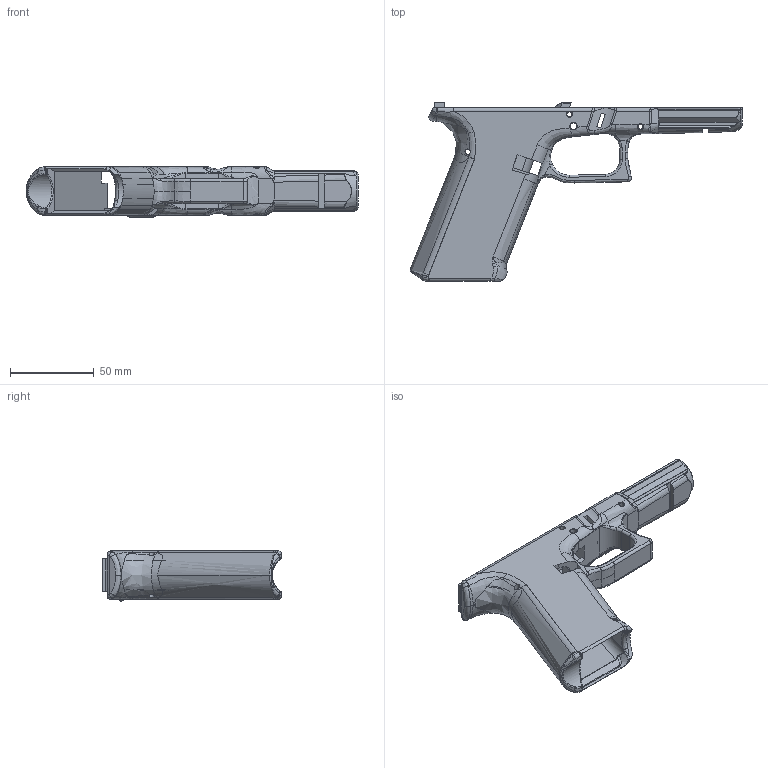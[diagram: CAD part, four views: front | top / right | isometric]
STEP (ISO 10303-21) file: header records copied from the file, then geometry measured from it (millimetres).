
FILE_DESCRIPTION(/* description */ (''),/* implementation_level */ '2;1');
FILE_NAME(/* name */ 'FMDA DD17.2 V1.4 G5Spring Frame.stp',/* time_stamp */ '2021-01-20T14:58:52-06:00',/* author */ ('johne'),/* organization */ (''),/* preprocessor_version */ 'ST-DEVELOPER v18',/* originating_system */ 'Autodesk Inventor 2020',/* authorisation */ '');
FILE_SCHEMA (('AUTOMOTIVE_DESIGN { 1 0 10303 214 3 1 1 }'));
Products named in the file (1): FMDA DD17.2 V1.4 Frame
Bounding box: 197.63 x 106.5 x 29.84 mm (x, y, z)
Volume: 86215.3 mm3; surface area: 46976.6 mm2
Topology: 1 solids, 3 shells, 631 faces, 1833 edges, 1176 vertices
Faces by surface type: bspline 289, plane 178, cylinder 121, torus 21, cone 12, sphere 10
Full cylindrical faces by diameter (mm): 2 x1, 3 x4, 3.2 x2, 3.81 x1, 4 x2
Entity records: 51301 total; most frequent: CARTESIAN_POINT 36483, ORIENTED_EDGE 3642, DIRECTION 2400, EDGE_CURVE 1821, VERTEX_POINT 1177, AXIS2_PLACEMENT_3D 875, LINE 650, VECTOR 650
